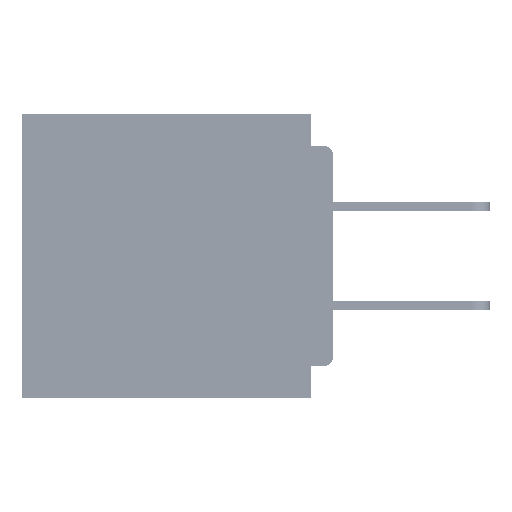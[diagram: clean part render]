
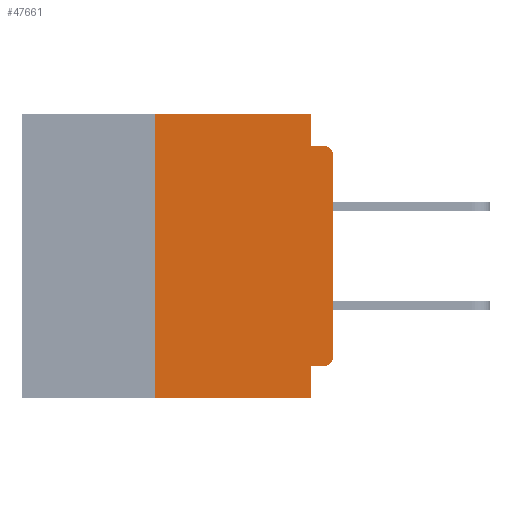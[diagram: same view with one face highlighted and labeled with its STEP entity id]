
A CAD part, left-side view. The second image highlights one B-rep face of the part: STEP entity #47661.
In plain terms, the highlighted planar face has unit normal (-1, 0, 0).
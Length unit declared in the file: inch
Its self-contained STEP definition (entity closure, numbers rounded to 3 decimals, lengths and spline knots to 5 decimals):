
#992 = ORIENTED_EDGE ( 'NONE', *, *, #14634, .T. ) ;
#1509 = DIRECTION ( 'NONE',  ( 0., 0., -1. ) ) ;
#1889 = DIRECTION ( 'NONE',  ( 0., 0., -1. ) ) ;
#2878 = CARTESIAN_POINT ( 'NONE',  ( 0., 0.015, -0.355 ) ) ;
#4687 = VECTOR ( 'NONE', #1889, 39.37008 ) ;
#5038 = DIRECTION ( 'NONE',  ( 1., 0., 0. ) ) ;
#6163 = CARTESIAN_POINT ( 'NONE',  ( 0., 0., -0.355 ) ) ;
#6928 = CARTESIAN_POINT ( 'NONE',  ( 0., 0.031, -0.4 ) ) ;
#7084 = VERTEX_POINT ( 'NONE', #44781 ) ;
#7162 = CARTESIAN_POINT ( 'NONE',  ( 0., 0.25, -0.4 ) ) ;
#7410 = LINE ( 'NONE', #54477, #34269 ) ;
#9940 = VECTOR ( 'NONE', #41193, 39.37008 ) ;
#10936 = EDGE_CURVE ( 'NONE', #41047, #47199, #26355, .T. ) ;
#12106 = VECTOR ( 'NONE', #27335, 39.37008 ) ;
#13638 = EDGE_CURVE ( 'NONE', #69396, #36462, #60339, .T. ) ;
#13738 = ORIENTED_EDGE ( 'NONE', *, *, #45605, .F. ) ;
#13870 = ORIENTED_EDGE ( 'NONE', *, *, #60665, .F. ) ;
#14634 = EDGE_CURVE ( 'NONE', #7084, #33246, #40115, .T. ) ;
#14790 = AXIS2_PLACEMENT_3D ( 'NONE', #26199, #5038, #42564 ) ;
#15255 = VERTEX_POINT ( 'NONE', #35724 ) ;
#15857 = VECTOR ( 'NONE', #38290, 39.37008 ) ;
#17382 = CARTESIAN_POINT ( 'NONE',  ( 0., 0.015, -0.06 ) ) ;
#19367 = ORIENTED_EDGE ( 'NONE', *, *, #32014, .T. ) ;
#20356 = CARTESIAN_POINT ( 'NONE',  ( 0., 0.031, -0.355 ) ) ;
#20655 = LINE ( 'NONE', #28675, #4687 ) ;
#21368 = CIRCLE ( 'NONE', #58719, 0.015 ) ;
#21901 = CARTESIAN_POINT ( 'NONE',  ( 0., 0., 0. ) ) ;
#22799 = DIRECTION ( 'NONE',  ( 0., 0., -1. ) ) ;
#26199 = CARTESIAN_POINT ( 'NONE',  ( 0., 0.437, 0. ) ) ;
#26265 = CARTESIAN_POINT ( 'NONE',  ( 0., 0.437, 0. ) ) ;
#26355 = LINE ( 'NONE', #21901, #12106 ) ;
#26514 = LINE ( 'NONE', #7162, #67603 ) ;
#27335 = DIRECTION ( 'NONE',  ( 0., 0., 1. ) ) ;
#28053 = LINE ( 'NONE', #26265, #69138 ) ;
#28675 = CARTESIAN_POINT ( 'NONE',  ( 0., 0.031, 0. ) ) ;
#30372 = ORIENTED_EDGE ( 'NONE', *, *, #31446, .F. ) ;
#30780 = CIRCLE ( 'NONE', #51690, 0.015 ) ;
#31446 = EDGE_CURVE ( 'NONE', #7084, #51654, #26514, .T. ) ;
#31641 = DIRECTION ( 'NONE',  ( 0., -1., 0. ) ) ;
#32014 = EDGE_CURVE ( 'NONE', #47199, #58675, #21368, .T. ) ;
#33246 = VERTEX_POINT ( 'NONE', #6928 ) ;
#33706 = DIRECTION ( 'NONE',  ( -1., 0., 0. ) ) ;
#34269 = VECTOR ( 'NONE', #59848, 39.37008 ) ;
#35610 = CARTESIAN_POINT ( 'NONE',  ( 0., 0.031, -0.045 ) ) ;
#35724 = CARTESIAN_POINT ( 'NONE',  ( 0., 0.031, 0. ) ) ;
#35808 = CARTESIAN_POINT ( 'NONE',  ( 0., 0.437, -0.4 ) ) ;
#36462 = VERTEX_POINT ( 'NONE', #20356 ) ;
#36767 = EDGE_CURVE ( 'NONE', #69396, #41047, #30780, .T. ) ;
#38101 = CARTESIAN_POINT ( 'NONE',  ( 0., 0., -0.34 ) ) ;
#38290 = DIRECTION ( 'NONE',  ( 0., 1., 0. ) ) ;
#39539 = ORIENTED_EDGE ( 'NONE', *, *, #13638, .F. ) ;
#40115 = LINE ( 'NONE', #35808, #9940 ) ;
#41047 = VERTEX_POINT ( 'NONE', #38101 ) ;
#41193 = DIRECTION ( 'NONE',  ( 0., -1., 0. ) ) ;
#42007 = LINE ( 'NONE', #68997, #52923 ) ;
#42264 = DIRECTION ( 'NONE',  ( 0., -1., 0. ) ) ;
#42564 = DIRECTION ( 'NONE',  ( 0., 0., -1. ) ) ;
#43218 = ORIENTED_EDGE ( 'NONE', *, *, #10936, .T. ) ;
#44781 = CARTESIAN_POINT ( 'NONE',  ( 0., 0.25, -0.4 ) ) ;
#45605 = EDGE_CURVE ( 'NONE', #15255, #46339, #20655, .T. ) ;
#46339 = VERTEX_POINT ( 'NONE', #35610 ) ;
#46957 = EDGE_LOOP ( 'NONE', ( #43218, #19367, #61568, #13738, #61216, #30372, #992, #13870, #39539, #55464 ) ) ;
#47199 = VERTEX_POINT ( 'NONE', #64148 ) ;
#47661 = ADVANCED_FACE ( 'NONE', ( #67523 ), #63959, .F. ) ;
#50044 = DIRECTION ( 'NONE',  ( 0., 0., 1. ) ) ;
#51654 = VERTEX_POINT ( 'NONE', #54832 ) ;
#51690 = AXIS2_PLACEMENT_3D ( 'NONE', #65831, #33706, #1509 ) ;
#52923 = VECTOR ( 'NONE', #42264, 39.37008 ) ;
#54085 = EDGE_CURVE ( 'NONE', #46339, #58675, #42007, .T. ) ;
#54477 = CARTESIAN_POINT ( 'NONE',  ( 0., 0.031, -0.4 ) ) ;
#54832 = CARTESIAN_POINT ( 'NONE',  ( 0., 0.25, 0. ) ) ;
#54932 = DIRECTION ( 'NONE',  ( -1., 0., 0. ) ) ;
#55464 = ORIENTED_EDGE ( 'NONE', *, *, #36767, .T. ) ;
#58498 = EDGE_CURVE ( 'NONE', #51654, #15255, #28053, .T. ) ;
#58675 = VERTEX_POINT ( 'NONE', #59771 ) ;
#58719 = AXIS2_PLACEMENT_3D ( 'NONE', #17382, #54932, #22799 ) ;
#59771 = CARTESIAN_POINT ( 'NONE',  ( 0., 0.015, -0.045 ) ) ;
#59848 = DIRECTION ( 'NONE',  ( 0., 0., -1. ) ) ;
#60339 = LINE ( 'NONE', #6163, #15857 ) ;
#60665 = EDGE_CURVE ( 'NONE', #36462, #33246, #7410, .T. ) ;
#61216 = ORIENTED_EDGE ( 'NONE', *, *, #58498, .F. ) ;
#61568 = ORIENTED_EDGE ( 'NONE', *, *, #54085, .F. ) ;
#63959 = PLANE ( 'NONE',  #14790 ) ;
#64148 = CARTESIAN_POINT ( 'NONE',  ( 0., 0., -0.06 ) ) ;
#65831 = CARTESIAN_POINT ( 'NONE',  ( 0., 0.015, -0.34 ) ) ;
#67523 = FACE_OUTER_BOUND ( 'NONE', #46957, .T. ) ;
#67603 = VECTOR ( 'NONE', #50044, 39.37008 ) ;
#68997 = CARTESIAN_POINT ( 'NONE',  ( 0., 0., -0.045 ) ) ;
#69138 = VECTOR ( 'NONE', #31641, 39.37008 ) ;
#69396 = VERTEX_POINT ( 'NONE', #2878 ) ;
